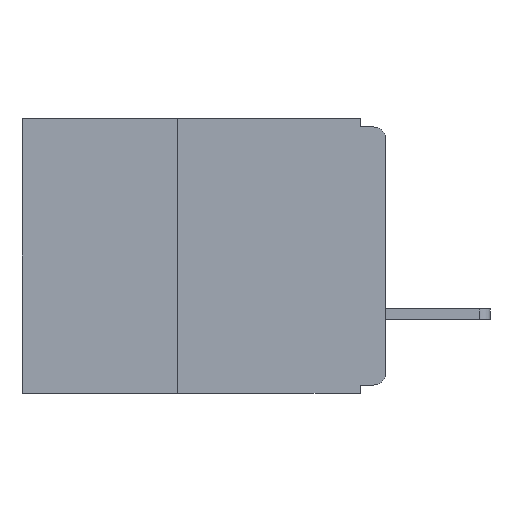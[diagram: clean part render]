
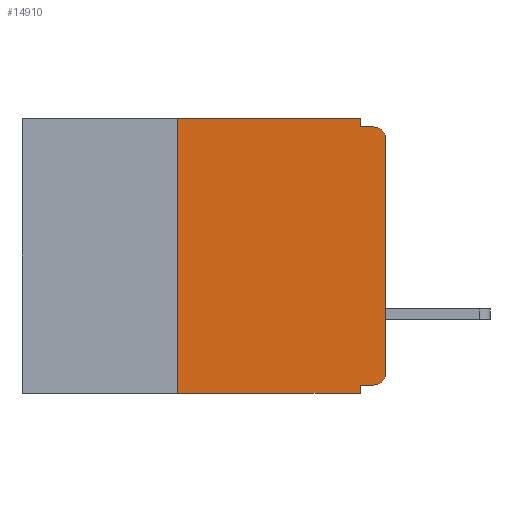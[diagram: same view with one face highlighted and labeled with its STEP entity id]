
A CAD part, left-side view. The second image highlights one B-rep face of the part: STEP entity #14910.
In plain terms, the highlighted planar face has unit normal (-1, 0, 0).
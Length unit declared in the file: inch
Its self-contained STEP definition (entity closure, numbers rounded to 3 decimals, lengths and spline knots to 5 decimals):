
#360 = CARTESIAN_POINT ( 'NONE',  ( 0., 0.031, -0.33 ) ) ;
#1283 = PLANE ( 'NONE',  #11792 ) ;
#1676 = CARTESIAN_POINT ( 'NONE',  ( 0., 0.437, -0.33 ) ) ;
#1943 = LINE ( 'NONE', #2773, #16347 ) ;
#2254 = CARTESIAN_POINT ( 'NONE',  ( 0., 0., -0.32 ) ) ;
#2337 = VERTEX_POINT ( 'NONE', #15447 ) ;
#2574 = VECTOR ( 'NONE', #12623, 39.37008 ) ;
#2773 = CARTESIAN_POINT ( 'NONE',  ( 0., 0.25, -0.33 ) ) ;
#2992 = CARTESIAN_POINT ( 'NONE',  ( 0., 0.015, -0.01 ) ) ;
#3234 = EDGE_CURVE ( 'NONE', #8661, #6824, #4610, .T. ) ;
#3436 = CARTESIAN_POINT ( 'NONE',  ( 0., 0.015, -0.025 ) ) ;
#3901 = VECTOR ( 'NONE', #18349, 39.37008 ) ;
#4183 = VERTEX_POINT ( 'NONE', #17271 ) ;
#4392 = EDGE_CURVE ( 'NONE', #21753, #2337, #8313, .T. ) ;
#4578 = CARTESIAN_POINT ( 'NONE',  ( 0., 0., 0. ) ) ;
#4610 = LINE ( 'NONE', #7558, #22299 ) ;
#4781 = CARTESIAN_POINT ( 'NONE',  ( 0., 0.015, -0.32 ) ) ;
#5094 = EDGE_CURVE ( 'NONE', #10186, #4183, #8027, .T. ) ;
#5294 = DIRECTION ( 'NONE',  ( 0., 0., -1. ) ) ;
#5351 = LINE ( 'NONE', #5557, #13892 ) ;
#5379 = EDGE_CURVE ( 'NONE', #10186, #7454, #1943, .T. ) ;
#5557 = CARTESIAN_POINT ( 'NONE',  ( 0., 0.437, 0. ) ) ;
#5653 = ORIENTED_EDGE ( 'NONE', *, *, #15384, .T. ) ;
#5677 = EDGE_CURVE ( 'NONE', #7454, #8661, #5351, .T. ) ;
#5966 = EDGE_CURVE ( 'NONE', #13997, #12064, #17674, .T. ) ;
#6436 = CARTESIAN_POINT ( 'NONE',  ( 0., 0.031, 0. ) ) ;
#6824 = VERTEX_POINT ( 'NONE', #7050 ) ;
#7050 = CARTESIAN_POINT ( 'NONE',  ( 0., 0.031, -0.01 ) ) ;
#7239 = ORIENTED_EDGE ( 'NONE', *, *, #3234, .F. ) ;
#7454 = VERTEX_POINT ( 'NONE', #8892 ) ;
#7558 = CARTESIAN_POINT ( 'NONE',  ( 0., 0.031, 0. ) ) ;
#7937 = DIRECTION ( 'NONE',  ( -1., 0., 0. ) ) ;
#8027 = LINE ( 'NONE', #1676, #12052 ) ;
#8313 = LINE ( 'NONE', #2254, #18019 ) ;
#8512 = ORIENTED_EDGE ( 'NONE', *, *, #21280, .T. ) ;
#8661 = VERTEX_POINT ( 'NONE', #6436 ) ;
#8892 = CARTESIAN_POINT ( 'NONE',  ( 0., 0.25, 0. ) ) ;
#8908 = ORIENTED_EDGE ( 'NONE', *, *, #5677, .F. ) ;
#9120 = CARTESIAN_POINT ( 'NONE',  ( 0., 0.25, -0.33 ) ) ;
#9468 = CARTESIAN_POINT ( 'NONE',  ( 0., 0., -0.01 ) ) ;
#10113 = DIRECTION ( 'NONE',  ( 1., 0., 0. ) ) ;
#10186 = VERTEX_POINT ( 'NONE', #9120 ) ;
#10193 = ORIENTED_EDGE ( 'NONE', *, *, #5966, .T. ) ;
#10976 = DIRECTION ( 'NONE',  ( 0., 0., -1. ) ) ;
#11120 = ORIENTED_EDGE ( 'NONE', *, *, #16750, .F. ) ;
#11166 = CARTESIAN_POINT ( 'NONE',  ( 0., 0., -0.025 ) ) ;
#11419 = ORIENTED_EDGE ( 'NONE', *, *, #4392, .F. ) ;
#11454 = DIRECTION ( 'NONE',  ( 0., 0., 1. ) ) ;
#11539 = EDGE_CURVE ( 'NONE', #6824, #18265, #16137, .T. ) ;
#11792 = AXIS2_PLACEMENT_3D ( 'NONE', #20422, #10113, #22091 ) ;
#12052 = VECTOR ( 'NONE', #12135, 39.37008 ) ;
#12064 = VERTEX_POINT ( 'NONE', #11166 ) ;
#12106 = VECTOR ( 'NONE', #21475, 39.37008 ) ;
#12135 = DIRECTION ( 'NONE',  ( 0., -1., 0. ) ) ;
#12623 = DIRECTION ( 'NONE',  ( 0., 0., -1. ) ) ;
#13233 = ORIENTED_EDGE ( 'NONE', *, *, #5379, .F. ) ;
#13892 = VECTOR ( 'NONE', #14054, 39.37008 ) ;
#13997 = VERTEX_POINT ( 'NONE', #19250 ) ;
#14054 = DIRECTION ( 'NONE',  ( 0., -1., 0. ) ) ;
#14389 = DIRECTION ( 'NONE',  ( 0., 1., 0. ) ) ;
#14468 = AXIS2_PLACEMENT_3D ( 'NONE', #3436, #15530, #5294 ) ;
#14910 = ADVANCED_FACE ( 'NONE', ( #22092 ), #1283, .F. ) ;
#15366 = ORIENTED_EDGE ( 'NONE', *, *, #5094, .T. ) ;
#15384 = EDGE_CURVE ( 'NONE', #21753, #13997, #18632, .T. ) ;
#15447 = CARTESIAN_POINT ( 'NONE',  ( 0., 0.031, -0.32 ) ) ;
#15530 = DIRECTION ( 'NONE',  ( -1., 0., 0. ) ) ;
#16137 = LINE ( 'NONE', #9468, #12106 ) ;
#16347 = VECTOR ( 'NONE', #11454, 39.37008 ) ;
#16750 = EDGE_CURVE ( 'NONE', #2337, #4183, #19376, .T. ) ;
#17271 = CARTESIAN_POINT ( 'NONE',  ( 0., 0.031, -0.33 ) ) ;
#17674 = LINE ( 'NONE', #4578, #3901 ) ;
#17729 = EDGE_LOOP ( 'NONE', ( #10193, #8512, #20302, #7239, #8908, #13233, #15366, #11120, #11419, #5653 ) ) ;
#18019 = VECTOR ( 'NONE', #14389, 39.37008 ) ;
#18235 = CARTESIAN_POINT ( 'NONE',  ( 0., 0.015, -0.305 ) ) ;
#18265 = VERTEX_POINT ( 'NONE', #2992 ) ;
#18349 = DIRECTION ( 'NONE',  ( 0., 0., 1. ) ) ;
#18632 = CIRCLE ( 'NONE', #19449, 0.015 ) ;
#18662 = CIRCLE ( 'NONE', #14468, 0.015 ) ;
#19250 = CARTESIAN_POINT ( 'NONE',  ( 0., 0., -0.305 ) ) ;
#19376 = LINE ( 'NONE', #360, #2574 ) ;
#19449 = AXIS2_PLACEMENT_3D ( 'NONE', #18235, #7937, #19973 ) ;
#19973 = DIRECTION ( 'NONE',  ( 0., 0., -1. ) ) ;
#20302 = ORIENTED_EDGE ( 'NONE', *, *, #11539, .F. ) ;
#20422 = CARTESIAN_POINT ( 'NONE',  ( 0., 0.437, 0. ) ) ;
#21280 = EDGE_CURVE ( 'NONE', #12064, #18265, #18662, .T. ) ;
#21475 = DIRECTION ( 'NONE',  ( 0., -1., 0. ) ) ;
#21753 = VERTEX_POINT ( 'NONE', #4781 ) ;
#22091 = DIRECTION ( 'NONE',  ( 0., 0., -1. ) ) ;
#22092 = FACE_OUTER_BOUND ( 'NONE', #17729, .T. ) ;
#22299 = VECTOR ( 'NONE', #10976, 39.37008 ) ;
